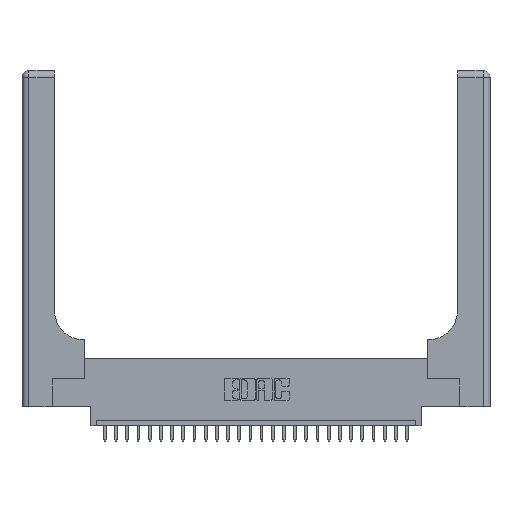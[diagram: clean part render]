
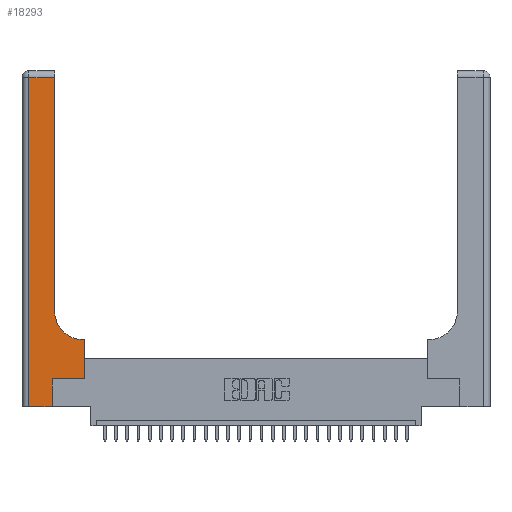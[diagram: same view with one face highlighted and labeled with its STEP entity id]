
A CAD part, top view. The second image highlights one B-rep face of the part: STEP entity #18293.
In plain terms, the highlighted planar face has unit normal (0, 0, 1).
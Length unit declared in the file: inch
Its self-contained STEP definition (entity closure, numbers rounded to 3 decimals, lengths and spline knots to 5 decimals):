
#158 = CARTESIAN_POINT ( 'NONE',  ( 0., 2.94, 0.37 ) ) ;
#1034 = CARTESIAN_POINT ( 'NONE',  ( 0.5415, 0.85, 0.37 ) ) ;
#2464 = DIRECTION ( 'NONE',  ( 1., 0., 0. ) ) ;
#2503 = LINE ( 'NONE', #26800, #13427 ) ;
#2670 = DIRECTION ( 'NONE',  ( 0., 1., 0. ) ) ;
#2790 = CARTESIAN_POINT ( 'NONE',  ( 0.5415, 0.6, 0.37 ) ) ;
#3255 = VERTEX_POINT ( 'NONE', #16959 ) ;
#4038 = CARTESIAN_POINT ( 'NONE',  ( 0.2915, 0.6, 0.37 ) ) ;
#4488 = VERTEX_POINT ( 'NONE', #21191 ) ;
#4715 = VECTOR ( 'NONE', #9314, 39.37008 ) ;
#4770 = VERTEX_POINT ( 'NONE', #2790 ) ;
#5385 = CARTESIAN_POINT ( 'NONE',  ( 0.2915, 2.94, 0.37 ) ) ;
#5544 = DIRECTION ( 'NONE',  ( 0., 0., -1. ) ) ;
#5918 = ORIENTED_EDGE ( 'NONE', *, *, #7373, .T. ) ;
#6190 = VERTEX_POINT ( 'NONE', #16410 ) ;
#6243 = DIRECTION ( 'NONE',  ( -1., 0., 0. ) ) ;
#7045 = CARTESIAN_POINT ( 'NONE',  ( 0.06, 3., 0.37 ) ) ;
#7373 = EDGE_CURVE ( 'NONE', #15116, #21327, #22341, .T. ) ;
#8269 = AXIS2_PLACEMENT_3D ( 'NONE', #1034, #5544, #22805 ) ;
#8509 = VECTOR ( 'NONE', #6243, 39.37008 ) ;
#8546 = EDGE_CURVE ( 'NONE', #6190, #26443, #2503, .T. ) ;
#8653 = CARTESIAN_POINT ( 'NONE',  ( 0.2915, 0.85, 0.37 ) ) ;
#9314 = DIRECTION ( 'NONE',  ( -1., 0., 0. ) ) ;
#10881 = VECTOR ( 'NONE', #17957, 39.37008 ) ;
#11050 = DIRECTION ( 'NONE',  ( 1., 0., 0. ) ) ;
#11192 = LINE ( 'NONE', #7045, #10881 ) ;
#11404 = EDGE_CURVE ( 'NONE', #3255, #4770, #16717, .T. ) ;
#11465 = CARTESIAN_POINT ( 'NONE',  ( 0.2915, 3., 0.37 ) ) ;
#11570 = ORIENTED_EDGE ( 'NONE', *, *, #15501, .T. ) ;
#12400 = EDGE_CURVE ( 'NONE', #21327, #21948, #19413, .T. ) ;
#12404 = VERTEX_POINT ( 'NONE', #25673 ) ;
#12716 = EDGE_LOOP ( 'NONE', ( #5918, #21751, #20187, #11570, #24063, #17803, #14692, #20031, #22880 ) ) ;
#12814 = EDGE_CURVE ( 'NONE', #21948, #4488, #11192, .T. ) ;
#12928 = PLANE ( 'NONE',  #13322 ) ;
#13322 = AXIS2_PLACEMENT_3D ( 'NONE', #17637, #15246, #28198 ) ;
#13427 = VECTOR ( 'NONE', #22311, 39.37008 ) ;
#14222 = DIRECTION ( 'NONE',  ( 0., 1., 0. ) ) ;
#14692 = ORIENTED_EDGE ( 'NONE', *, *, #23829, .T. ) ;
#15003 = LINE ( 'NONE', #19717, #23161 ) ;
#15116 = VERTEX_POINT ( 'NONE', #8653 ) ;
#15246 = DIRECTION ( 'NONE',  ( 0., 0., -1. ) ) ;
#15501 = EDGE_CURVE ( 'NONE', #4488, #6190, #18259, .T. ) ;
#16354 = FACE_OUTER_BOUND ( 'NONE', #12716, .T. ) ;
#16406 = CARTESIAN_POINT ( 'NONE',  ( 0., 0., 0.37 ) ) ;
#16410 = CARTESIAN_POINT ( 'NONE',  ( 0.269, 0., 0.37 ) ) ;
#16717 = LINE ( 'NONE', #4038, #8509 ) ;
#16959 = CARTESIAN_POINT ( 'NONE',  ( 0.5585, 0.6, 0.37 ) ) ;
#17637 = CARTESIAN_POINT ( 'NONE',  ( 0., 3., 0.37 ) ) ;
#17803 = ORIENTED_EDGE ( 'NONE', *, *, #18321, .T. ) ;
#17911 = CARTESIAN_POINT ( 'NONE',  ( 0.06, 2.94, 0.37 ) ) ;
#17957 = DIRECTION ( 'NONE',  ( 0., -1., 0. ) ) ;
#18259 = LINE ( 'NONE', #16406, #18576 ) ;
#18293 = ADVANCED_FACE ( 'NONE', ( #16354 ), #12928, .F. ) ;
#18321 = EDGE_CURVE ( 'NONE', #26443, #12404, #15003, .T. ) ;
#18576 = VECTOR ( 'NONE', #2464, 39.37008 ) ;
#19065 = CIRCLE ( 'NONE', #8269, 0.25 ) ;
#19413 = LINE ( 'NONE', #158, #4715 ) ;
#19717 = CARTESIAN_POINT ( 'NONE',  ( 0.269, 0.25, 0.37 ) ) ;
#20031 = ORIENTED_EDGE ( 'NONE', *, *, #11404, .T. ) ;
#20187 = ORIENTED_EDGE ( 'NONE', *, *, #12814, .T. ) ;
#20970 = VECTOR ( 'NONE', #14222, 39.37008 ) ;
#21191 = CARTESIAN_POINT ( 'NONE',  ( 0.06, 0., 0.37 ) ) ;
#21327 = VERTEX_POINT ( 'NONE', #5385 ) ;
#21751 = ORIENTED_EDGE ( 'NONE', *, *, #12400, .T. ) ;
#21948 = VERTEX_POINT ( 'NONE', #17911 ) ;
#22031 = EDGE_CURVE ( 'NONE', #4770, #15116, #19065, .T. ) ;
#22311 = DIRECTION ( 'NONE',  ( 0., 1., 0. ) ) ;
#22341 = LINE ( 'NONE', #11465, #20970 ) ;
#22342 = LINE ( 'NONE', #22612, #24738 ) ;
#22612 = CARTESIAN_POINT ( 'NONE',  ( 0.5585, 0.25, 0.37 ) ) ;
#22805 = DIRECTION ( 'NONE',  ( 1., 0., 0. ) ) ;
#22880 = ORIENTED_EDGE ( 'NONE', *, *, #22031, .T. ) ;
#23161 = VECTOR ( 'NONE', #11050, 39.37008 ) ;
#23540 = CARTESIAN_POINT ( 'NONE',  ( 0.269, 0.25, 0.37 ) ) ;
#23829 = EDGE_CURVE ( 'NONE', #12404, #3255, #22342, .T. ) ;
#24063 = ORIENTED_EDGE ( 'NONE', *, *, #8546, .T. ) ;
#24738 = VECTOR ( 'NONE', #2670, 39.37008 ) ;
#25673 = CARTESIAN_POINT ( 'NONE',  ( 0.5585, 0.25, 0.37 ) ) ;
#26443 = VERTEX_POINT ( 'NONE', #23540 ) ;
#26800 = CARTESIAN_POINT ( 'NONE',  ( 0.269, 0., 0.37 ) ) ;
#28198 = DIRECTION ( 'NONE',  ( -1., 0., 0. ) ) ;
